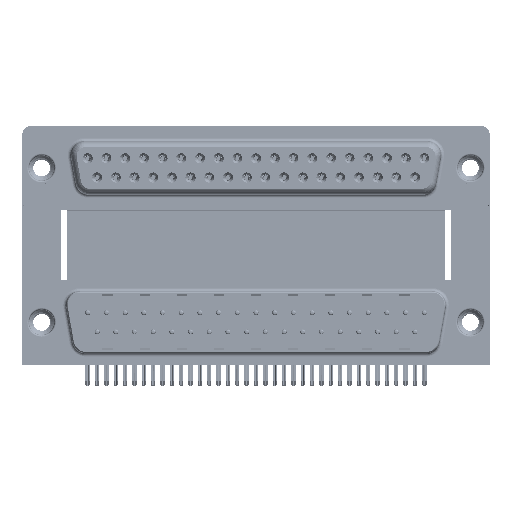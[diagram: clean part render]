
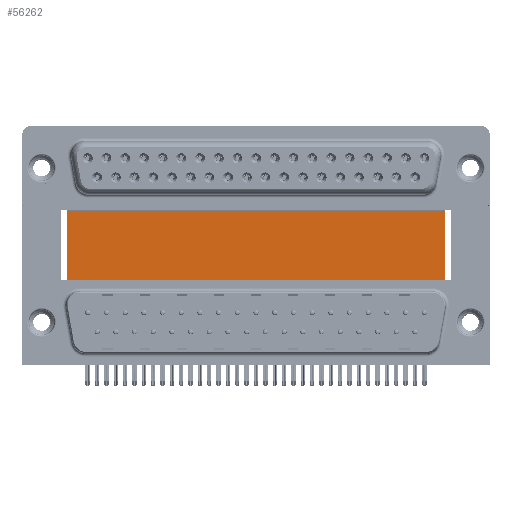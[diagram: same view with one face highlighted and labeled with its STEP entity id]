
A CAD part, top view. The second image highlights one B-rep face of the part: STEP entity #56262.
In plain terms, the highlighted planar face has unit normal (0, 0, 1).
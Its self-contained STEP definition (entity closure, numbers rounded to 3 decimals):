
#1463 = VECTOR ( 'NONE', #27559, 1000. ) ;
#1807 = DIRECTION ( 'NONE',  ( 1., 0., 0. ) ) ;
#2782 = LINE ( 'NONE', #55215, #36929 ) ;
#3194 = VERTEX_POINT ( 'NONE', #58467 ) ;
#4081 = EDGE_CURVE ( 'NONE', #26222, #54709, #54234, .T. ) ;
#6195 = DIRECTION ( 'NONE',  ( -1., 0., 0. ) ) ;
#8067 = LINE ( 'NONE', #35099, #51837 ) ;
#13206 = CARTESIAN_POINT ( 'NONE',  ( 59.71, -3.735, -12. ) ) ;
#17932 = EDGE_CURVE ( 'NONE', #26222, #3194, #48112, .T. ) ;
#21304 = CARTESIAN_POINT ( 'NONE',  ( 59.71, 16.585, -12. ) ) ;
#26222 = VERTEX_POINT ( 'NONE', #30535 ) ;
#26556 = CARTESIAN_POINT ( 'NONE',  ( 3.79, 16.585, -12. ) ) ;
#27421 = DIRECTION ( 'NONE',  ( 0., 0., -1. ) ) ;
#27559 = DIRECTION ( 'NONE',  ( 0., -1., 0. ) ) ;
#28209 = ORIENTED_EDGE ( 'NONE', *, *, #4081, .F. ) ;
#30535 = CARTESIAN_POINT ( 'NONE',  ( 3.79, 16.585, -12. ) ) ;
#31214 = VERTEX_POINT ( 'NONE', #13206 ) ;
#31525 = EDGE_LOOP ( 'NONE', ( #63881, #39507, #28209, #34645 ) ) ;
#32253 = FACE_OUTER_BOUND ( 'NONE', #31525, .T. ) ;
#34645 = ORIENTED_EDGE ( 'NONE', *, *, #17932, .T. ) ;
#35099 = CARTESIAN_POINT ( 'NONE',  ( 3.79, -3.735, -12. ) ) ;
#36929 = VECTOR ( 'NONE', #65796, 1000. ) ;
#39507 = ORIENTED_EDGE ( 'NONE', *, *, #62308, .F. ) ;
#39562 = DIRECTION ( 'NONE',  ( 1., 0., 0. ) ) ;
#46170 = AXIS2_PLACEMENT_3D ( 'NONE', #57616, #27421, #6195 ) ;
#48112 = LINE ( 'NONE', #26556, #1463 ) ;
#48418 = CARTESIAN_POINT ( 'NONE',  ( 3.79, 16.585, -12. ) ) ;
#51837 = VECTOR ( 'NONE', #39562, 1000. ) ;
#53141 = PLANE ( 'NONE',  #46170 ) ;
#53983 = EDGE_CURVE ( 'NONE', #3194, #31214, #8067, .T. ) ;
#54234 = LINE ( 'NONE', #48418, #66864 ) ;
#54709 = VERTEX_POINT ( 'NONE', #21304 ) ;
#55215 = CARTESIAN_POINT ( 'NONE',  ( 59.71, 16.585, -12. ) ) ;
#56262 = ADVANCED_FACE ( 'NONE', ( #32253 ), #53141, .F. ) ;
#57616 = CARTESIAN_POINT ( 'NONE',  ( 3.79, 16.585, -12. ) ) ;
#58467 = CARTESIAN_POINT ( 'NONE',  ( 3.79, -3.735, -12. ) ) ;
#62308 = EDGE_CURVE ( 'NONE', #54709, #31214, #2782, .T. ) ;
#63881 = ORIENTED_EDGE ( 'NONE', *, *, #53983, .T. ) ;
#65796 = DIRECTION ( 'NONE',  ( 0., -1., 0. ) ) ;
#66864 = VECTOR ( 'NONE', #1807, 1000. ) ;
